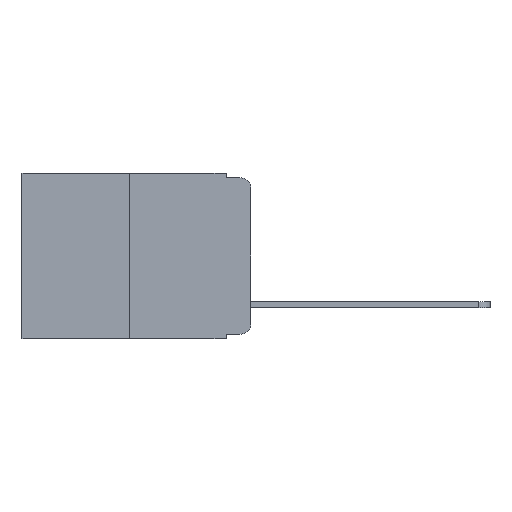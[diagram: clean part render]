
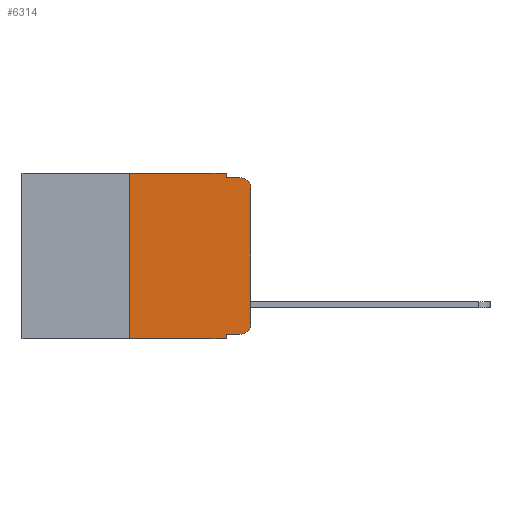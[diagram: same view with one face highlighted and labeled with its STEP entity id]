
A CAD part, left-side view. The second image highlights one B-rep face of the part: STEP entity #6314.
In plain terms, the highlighted planar face has unit normal (-1, 0, 0).
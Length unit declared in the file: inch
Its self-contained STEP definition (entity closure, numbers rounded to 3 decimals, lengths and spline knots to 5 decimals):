
#109 = EDGE_CURVE ( 'NONE', #4365, #9203, #9992, .T. ) ;
#265 = EDGE_CURVE ( 'NONE', #13240, #8292, #4773, .T. ) ;
#367 = DIRECTION ( 'NONE',  ( 0., 0., -1. ) ) ;
#756 = VECTOR ( 'NONE', #9167, 39.37008 ) ;
#783 = VERTEX_POINT ( 'NONE', #8089 ) ;
#1219 = CARTESIAN_POINT ( 'NONE',  ( 0., 0.25, 0. ) ) ;
#1694 = CARTESIAN_POINT ( 'NONE',  ( 0., 0., -0.313 ) ) ;
#2312 = AXIS2_PLACEMENT_3D ( 'NONE', #12968, #6976, #6839 ) ;
#2576 = CARTESIAN_POINT ( 'NONE',  ( 0., 0.051, -0.333 ) ) ;
#2735 = CARTESIAN_POINT ( 'NONE',  ( 0., 0.02, -0.333 ) ) ;
#2757 = LINE ( 'NONE', #3145, #10087 ) ;
#2778 = CARTESIAN_POINT ( 'NONE',  ( 0., 0.051, 0. ) ) ;
#2805 = ORIENTED_EDGE ( 'NONE', *, *, #265, .T. ) ;
#2872 = DIRECTION ( 'NONE',  ( 0., 0., -1. ) ) ;
#3145 = CARTESIAN_POINT ( 'NONE',  ( 0., 0.473, -0.343 ) ) ;
#3300 = FACE_OUTER_BOUND ( 'NONE', #5583, .T. ) ;
#3535 = VERTEX_POINT ( 'NONE', #10159 ) ;
#4002 = ORIENTED_EDGE ( 'NONE', *, *, #109, .F. ) ;
#4239 = VECTOR ( 'NONE', #9673, 39.37008 ) ;
#4282 = VECTOR ( 'NONE', #2872, 39.37008 ) ;
#4308 = EDGE_CURVE ( 'NONE', #8320, #11323, #10436, .T. ) ;
#4365 = VERTEX_POINT ( 'NONE', #7570 ) ;
#4384 = VECTOR ( 'NONE', #7529, 39.37008 ) ;
#4444 = VECTOR ( 'NONE', #8555, 39.37008 ) ;
#4773 = LINE ( 'NONE', #5390, #4444 ) ;
#4972 = CARTESIAN_POINT ( 'NONE',  ( 0., 0.25, -0.343 ) ) ;
#5390 = CARTESIAN_POINT ( 'NONE',  ( 0., 0., 0. ) ) ;
#5462 = ORIENTED_EDGE ( 'NONE', *, *, #8526, .T. ) ;
#5477 = CARTESIAN_POINT ( 'NONE',  ( 0., 0.02, -0.313 ) ) ;
#5583 = EDGE_LOOP ( 'NONE', ( #2805, #10037, #4002, #8275, #10176, #8305, #5462, #11513, #9378, #12255 ) ) ;
#5829 = PLANE ( 'NONE',  #2312 ) ;
#6314 = ADVANCED_FACE ( 'NONE', ( #3300 ), #5829, .F. ) ;
#6351 = DIRECTION ( 'NONE',  ( 0., -1., 0. ) ) ;
#6839 = DIRECTION ( 'NONE',  ( 0., 0., -1. ) ) ;
#6943 = VECTOR ( 'NONE', #12102, 39.37008 ) ;
#6976 = DIRECTION ( 'NONE',  ( 1., 0., 0. ) ) ;
#6991 = CARTESIAN_POINT ( 'NONE',  ( 0., 0.051, -0.333 ) ) ;
#7046 = VERTEX_POINT ( 'NONE', #6991 ) ;
#7291 = CARTESIAN_POINT ( 'NONE',  ( 0., 0.02, -0.01 ) ) ;
#7465 = VECTOR ( 'NONE', #6351, 39.37008 ) ;
#7522 = CARTESIAN_POINT ( 'NONE',  ( 0., 0.051, -0.01 ) ) ;
#7529 = DIRECTION ( 'NONE',  ( 0., 0., 1. ) ) ;
#7570 = CARTESIAN_POINT ( 'NONE',  ( 0., 0.051, -0.01 ) ) ;
#7809 = CARTESIAN_POINT ( 'NONE',  ( 0., 0.473, 0. ) ) ;
#7821 = EDGE_CURVE ( 'NONE', #7046, #13137, #13001, .T. ) ;
#7985 = CARTESIAN_POINT ( 'NONE',  ( 0., 0., -0.03 ) ) ;
#8089 = CARTESIAN_POINT ( 'NONE',  ( 0., 0.051, -0.343 ) ) ;
#8116 = CIRCLE ( 'NONE', #9701, 0.02 ) ;
#8155 = AXIS2_PLACEMENT_3D ( 'NONE', #11820, #9732, #8763 ) ;
#8241 = CIRCLE ( 'NONE', #8155, 0.02 ) ;
#8275 = ORIENTED_EDGE ( 'NONE', *, *, #13189, .F. ) ;
#8292 = VERTEX_POINT ( 'NONE', #7985 ) ;
#8305 = ORIENTED_EDGE ( 'NONE', *, *, #4308, .F. ) ;
#8320 = VERTEX_POINT ( 'NONE', #4972 ) ;
#8526 = EDGE_CURVE ( 'NONE', #8320, #783, #2757, .T. ) ;
#8555 = DIRECTION ( 'NONE',  ( 0., 0., 1. ) ) ;
#8763 = DIRECTION ( 'NONE',  ( 0., 0., -1. ) ) ;
#9167 = DIRECTION ( 'NONE',  ( 0., 0., -1. ) ) ;
#9203 = VERTEX_POINT ( 'NONE', #7291 ) ;
#9378 = ORIENTED_EDGE ( 'NONE', *, *, #7821, .T. ) ;
#9392 = LINE ( 'NONE', #10000, #756 ) ;
#9673 = DIRECTION ( 'NONE',  ( 0., -1., 0. ) ) ;
#9674 = LINE ( 'NONE', #7809, #6943 ) ;
#9701 = AXIS2_PLACEMENT_3D ( 'NONE', #5477, #12595, #367 ) ;
#9732 = DIRECTION ( 'NONE',  ( -1., 0., 0. ) ) ;
#9845 = LINE ( 'NONE', #2778, #4282 ) ;
#9992 = LINE ( 'NONE', #7522, #7465 ) ;
#10000 = CARTESIAN_POINT ( 'NONE',  ( 0., 0.051, 0. ) ) ;
#10037 = ORIENTED_EDGE ( 'NONE', *, *, #11733, .T. ) ;
#10087 = VECTOR ( 'NONE', #12075, 39.37008 ) ;
#10159 = CARTESIAN_POINT ( 'NONE',  ( 0., 0.051, 0. ) ) ;
#10176 = ORIENTED_EDGE ( 'NONE', *, *, #12244, .F. ) ;
#10388 = EDGE_CURVE ( 'NONE', #13137, #13240, #8116, .T. ) ;
#10436 = LINE ( 'NONE', #1219, #4384 ) ;
#10799 = EDGE_CURVE ( 'NONE', #7046, #783, #9392, .T. ) ;
#11323 = VERTEX_POINT ( 'NONE', #13182 ) ;
#11513 = ORIENTED_EDGE ( 'NONE', *, *, #10799, .F. ) ;
#11733 = EDGE_CURVE ( 'NONE', #8292, #9203, #8241, .T. ) ;
#11820 = CARTESIAN_POINT ( 'NONE',  ( 0., 0.02, -0.03 ) ) ;
#12075 = DIRECTION ( 'NONE',  ( 0., -1., 0. ) ) ;
#12102 = DIRECTION ( 'NONE',  ( 0., -1., 0. ) ) ;
#12244 = EDGE_CURVE ( 'NONE', #11323, #3535, #9674, .T. ) ;
#12255 = ORIENTED_EDGE ( 'NONE', *, *, #10388, .T. ) ;
#12595 = DIRECTION ( 'NONE',  ( -1., 0., 0. ) ) ;
#12968 = CARTESIAN_POINT ( 'NONE',  ( 0., 0.473, 0. ) ) ;
#13001 = LINE ( 'NONE', #2576, #4239 ) ;
#13137 = VERTEX_POINT ( 'NONE', #2735 ) ;
#13182 = CARTESIAN_POINT ( 'NONE',  ( 0., 0.25, 0. ) ) ;
#13189 = EDGE_CURVE ( 'NONE', #3535, #4365, #9845, .T. ) ;
#13240 = VERTEX_POINT ( 'NONE', #1694 ) ;
